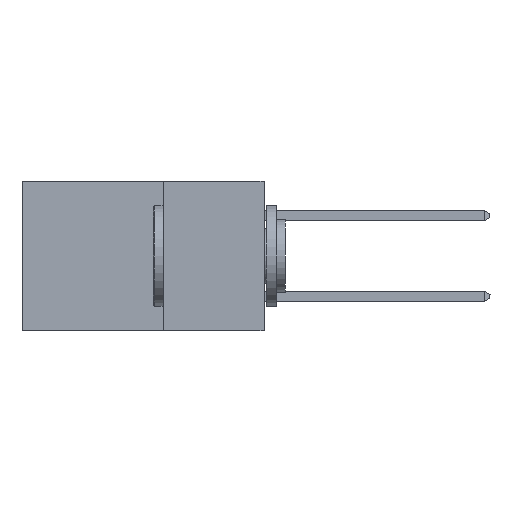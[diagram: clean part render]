
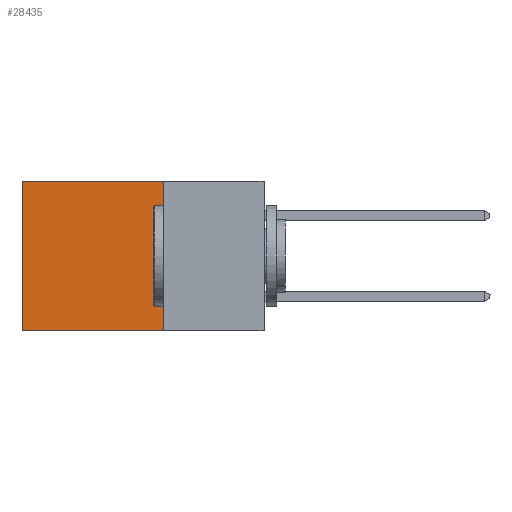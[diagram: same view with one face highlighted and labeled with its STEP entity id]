
A CAD part, left-side view. The second image highlights one B-rep face of the part: STEP entity #28435.
In plain terms, the highlighted planar face has unit normal (-1, 0, 0).
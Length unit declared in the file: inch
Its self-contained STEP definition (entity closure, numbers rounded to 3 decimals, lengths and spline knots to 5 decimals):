
#997 = VECTOR ( 'NONE', #9287, 39.37008 ) ;
#1490 = DIRECTION ( 'NONE',  ( 1., 0., 0. ) ) ;
#4055 = VERTEX_POINT ( 'NONE', #26074 ) ;
#4070 = ORIENTED_EDGE ( 'NONE', *, *, #17603, .F. ) ;
#4197 = ORIENTED_EDGE ( 'NONE', *, *, #28656, .T. ) ;
#4915 = VECTOR ( 'NONE', #11546, 39.37008 ) ;
#6169 = VERTEX_POINT ( 'NONE', #14363 ) ;
#6355 = PLANE ( 'NONE',  #10474 ) ;
#8171 = DIRECTION ( 'NONE',  ( 0., 0., -1. ) ) ;
#9149 = ORIENTED_EDGE ( 'NONE', *, *, #24799, .T. ) ;
#9287 = DIRECTION ( 'NONE',  ( 0., 0., -1. ) ) ;
#9372 = DIRECTION ( 'NONE',  ( 0., 1., 0. ) ) ;
#10474 = AXIS2_PLACEMENT_3D ( 'NONE', #11248, #1490, #30284 ) ;
#11248 = CARTESIAN_POINT ( 'NONE',  ( 0.298, 0.25, 0. ) ) ;
#11409 = LINE ( 'NONE', #30383, #13638 ) ;
#11546 = DIRECTION ( 'NONE',  ( 0., 1., 0. ) ) ;
#12837 = EDGE_CURVE ( 'NONE', #4055, #27559, #17796, .T. ) ;
#13638 = VECTOR ( 'NONE', #9372, 39.37008 ) ;
#13685 = VERTEX_POINT ( 'NONE', #16128 ) ;
#14031 = CARTESIAN_POINT ( 'NONE',  ( 0.298, 0.25, -0.37 ) ) ;
#14363 = CARTESIAN_POINT ( 'NONE',  ( 0.298, 0.6, 0. ) ) ;
#14855 = EDGE_LOOP ( 'NONE', ( #9149, #4070, #28404, #4197 ) ) ;
#15146 = CARTESIAN_POINT ( 'NONE',  ( 0.298, 0.25, -0.37 ) ) ;
#15656 = CARTESIAN_POINT ( 'NONE',  ( 0.298, 0.25, 0. ) ) ;
#16128 = CARTESIAN_POINT ( 'NONE',  ( 0.298, 0.6, -0.37 ) ) ;
#16221 = LINE ( 'NONE', #27391, #997 ) ;
#17603 = EDGE_CURVE ( 'NONE', #27559, #13685, #30093, .T. ) ;
#17796 = LINE ( 'NONE', #15656, #26325 ) ;
#23663 = FACE_OUTER_BOUND ( 'NONE', #14855, .T. ) ;
#24799 = EDGE_CURVE ( 'NONE', #6169, #13685, #16221, .T. ) ;
#26074 = CARTESIAN_POINT ( 'NONE',  ( 0.298, 0.25, 0. ) ) ;
#26325 = VECTOR ( 'NONE', #8171, 39.37008 ) ;
#27391 = CARTESIAN_POINT ( 'NONE',  ( 0.298, 0.6, 0. ) ) ;
#27559 = VERTEX_POINT ( 'NONE', #15146 ) ;
#28404 = ORIENTED_EDGE ( 'NONE', *, *, #12837, .F. ) ;
#28435 = ADVANCED_FACE ( 'NONE', ( #23663 ), #6355, .F. ) ;
#28656 = EDGE_CURVE ( 'NONE', #4055, #6169, #11409, .T. ) ;
#30093 = LINE ( 'NONE', #14031, #4915 ) ;
#30284 = DIRECTION ( 'NONE',  ( 0., 0., -1. ) ) ;
#30383 = CARTESIAN_POINT ( 'NONE',  ( 0.298, 0.25, 0. ) ) ;
